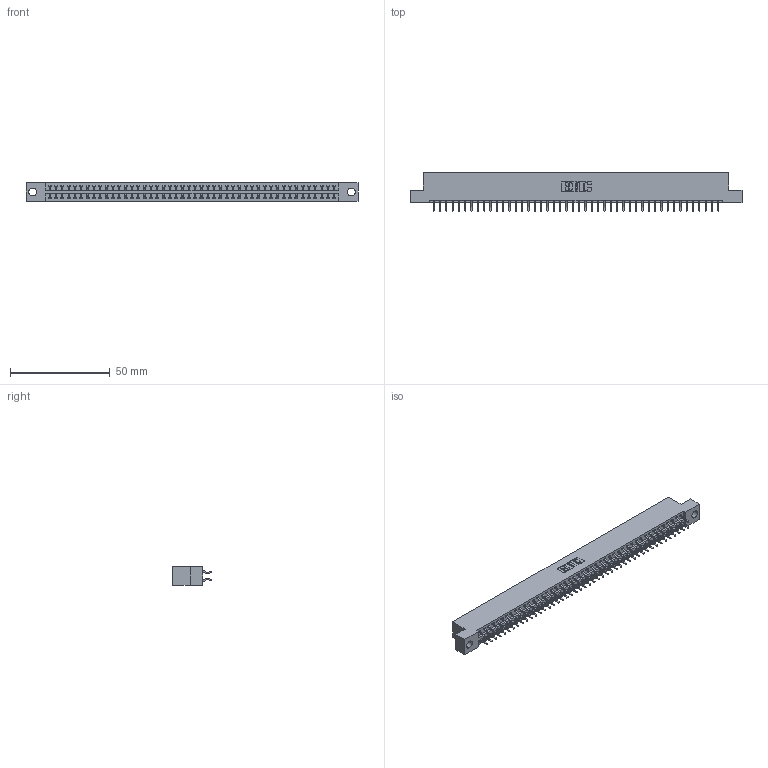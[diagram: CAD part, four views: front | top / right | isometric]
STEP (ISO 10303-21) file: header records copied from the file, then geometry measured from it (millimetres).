
FILE_DESCRIPTION (( 'STEP AP203' ), '1' );
FILE_NAME ('346-092-556-204.STEP', '2022-05-26T07:56:33', ( '' ), ( '' ), 'SwSTEP 2.0', 'SolidWorks 2020', '' );
FILE_SCHEMA (( 'CONFIG_CONTROL_DESIGN' ));
Length unit declared in the file: inch
Products named in the file (3): 345-292-001_556 Tail; 346-092-556-204; 346 Part_Flush Mounting Lugs - 0.156 Dia-TH
Assembly tree (93 placements, depth 2):
  346-092-556-204
    346 Part_Flush Mounting Lugs - 0.156 Dia-TH
    345-292-001_556 Tail  x92
Bounding box: 166.62 x 19.57 x 9.4 mm (x, y, z)
Volume: 16169.4 mm3; surface area: 22051.2 mm2
Topology: 93 solids, 93 shells, 5472 faces, 16281 edges, 10730 vertices
Faces by surface type: plane 3678, cylinder 1794
Entity records: 30121 total; most frequent: CARTESIAN_POINT 4978, ORIENTED_EDGE 4898, DIRECTION 4425, EDGE_CURVE 2449, VECTOR 2125, LINE 2125, VERTEX_POINT 1630, AXIS2_PLACEMENT_3D 1150
